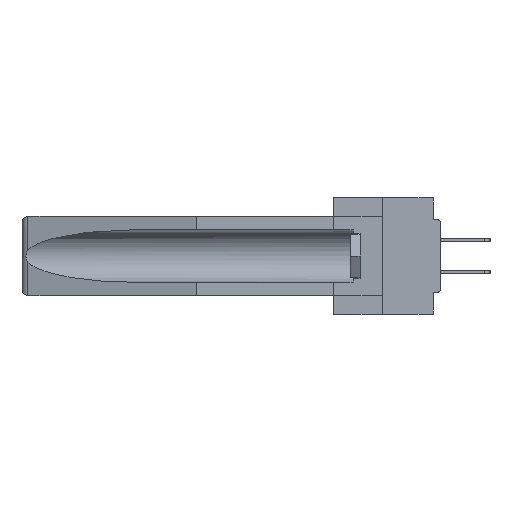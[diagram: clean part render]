
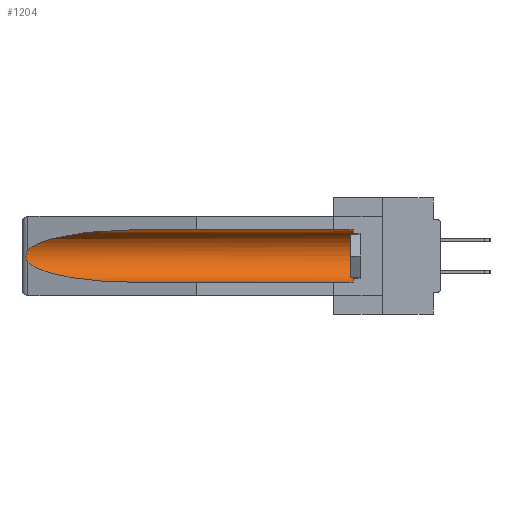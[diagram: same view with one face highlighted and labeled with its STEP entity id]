
A CAD part, left-side view. The second image highlights one B-rep face of the part: STEP entity #1204.
In plain terms, the highlighted cylindrical face has radius 2.857 mm (diameter 5.715 mm), a partial arc.
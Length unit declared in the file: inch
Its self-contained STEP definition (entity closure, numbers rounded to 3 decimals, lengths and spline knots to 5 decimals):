
#48 = CARTESIAN_POINT ( 'NONE',  ( 0.155, -0.30754, -0.1715 ) ) ;
#313 = CARTESIAN_POINT ( 'NONE',  ( 0.25451, 1.48313, -0.09465 ) ) ;
#1204 = ADVANCED_FACE ( 'NONE', ( #12092 ), #30902, .F. ) ;
#1375 = LINE ( 'NONE', #9870, #32835 ) ;
#2094 = EDGE_CURVE ( 'NONE', #26790, #12934, #27279, .T. ) ;
#2748 = B_SPLINE_CURVE_WITH_KNOTS ( 'NONE', 3,
 ( #4657, #32740, #17219, #38463, #13721, #35598, #35867, #26544, #13847, #10886 ),
 .UNSPECIFIED., .F., .F.,
 ( 4, 2, 2, 2, 4 ),
 ( 0., 0.00029, 0.00058, 0.00087, 0.00117 ),
 .UNSPECIFIED. ) ;
#2860 = CARTESIAN_POINT ( 'NONE',  ( 0.155, 0.126, -0.1715 ) ) ;
#3675 = AXIS2_PLACEMENT_3D ( 'NONE', #2860, #9345, #18841 ) ;
#4394 = CARTESIAN_POINT ( 'NONE',  ( 0.21114, 1.30732, -0.284 ) ) ;
#4505 = VERTEX_POINT ( 'NONE', #13082 ) ;
#4657 = CARTESIAN_POINT ( 'NONE',  ( 0.26537, 1.52718, -0.14972 ) ) ;
#6029 = ORIENTED_EDGE ( 'NONE', *, *, #30723, .T. ) ;
#6275 = CIRCLE ( 'NONE', #3675, 0.1125 ) ;
#6322 = CARTESIAN_POINT ( 'NONE',  ( 0.21114, 1.30732, -0.059 ) ) ;
#7328 = CARTESIAN_POINT ( 'NONE',  ( 0.26537, 1.52718, -0.14972 ) ) ;
#9345 = DIRECTION ( 'NONE',  ( 0., -1., 0. ) ) ;
#9870 = CARTESIAN_POINT ( 'NONE',  ( 0.155, -0.30754, -0.284 ) ) ;
#10499 = VERTEX_POINT ( 'NONE', #36795 ) ;
#10886 = CARTESIAN_POINT ( 'NONE',  ( 0.26537, 1.52718, -0.19328 ) ) ;
#11142 = ORIENTED_EDGE ( 'NONE', *, *, #31117, .T. ) ;
#11309 = VERTEX_POINT ( 'NONE', #14809 ) ;
#12092 = FACE_OUTER_BOUND ( 'NONE', #18877, .T. ) ;
#12934 = VERTEX_POINT ( 'NONE', #7328 ) ;
#13082 = CARTESIAN_POINT ( 'NONE',  ( 0.155, 1.07973, -0.284 ) ) ;
#13721 = CARTESIAN_POINT ( 'NONE',  ( 0.2675, 1.53308, -0.16763 ) ) ;
#13847 = CARTESIAN_POINT ( 'NONE',  ( 0.26597, 1.5296, -0.19026 ) ) ;
#14682 = EDGE_CURVE ( 'NONE', #34576, #10499, #6275, .T. ) ;
#14809 = CARTESIAN_POINT ( 'NONE',  ( 0.26537, 1.52718, -0.19328 ) ) ;
#15111 = DIRECTION ( 'NONE',  ( 0., 1., 0. ) ) ;
#17219 = CARTESIAN_POINT ( 'NONE',  ( 0.26654, 1.53092, -0.15636 ) ) ;
#18563 = LINE ( 'NONE', #27110, #19543 ) ;
#18841 = DIRECTION ( 'NONE',  ( 0., 0., 1. ) ) ;
#18877 = EDGE_LOOP ( 'NONE', ( #31115, #11142, #29495, #29835, #39743, #6029 ) ) ;
#19543 = VECTOR ( 'NONE', #27510, 39.37008 ) ;
#20088 = CARTESIAN_POINT ( 'NONE',  ( 0.155, 1.07973, -0.284 ) ) ;
#22238 = AXIS2_PLACEMENT_3D ( 'NONE', #48, #15111, #27399 ) ;
#25894 = CARTESIAN_POINT ( 'NONE',  ( 0.155, 1.07973, -0.059 ) ) ;
#26544 = CARTESIAN_POINT ( 'NONE',  ( 0.26655, 1.53094, -0.18657 ) ) ;
#26790 = VERTEX_POINT ( 'NONE', #38608 ) ;
#27110 = CARTESIAN_POINT ( 'NONE',  ( 0.155, -0.30754, -0.059 ) ) ;
#27279 =( BOUNDED_CURVE ( )  B_SPLINE_CURVE ( 3, ( #25894, #6322, #313, #40100 ),
 .UNSPECIFIED., .F., .F. ) 
 B_SPLINE_CURVE_WITH_KNOTS ( ( 4, 4 ),
 ( 4.71239, 6.08839 ),
 .UNSPECIFIED. ) 
 CURVE ( )  GEOMETRIC_REPRESENTATION_ITEM ( )  RATIONAL_B_SPLINE_CURVE ( ( 1., 0.848, 0.848, 1. ) ) 
 REPRESENTATION_ITEM ( '' )  );
#27399 = DIRECTION ( 'NONE',  ( 0., 0., 1. ) ) ;
#27510 = DIRECTION ( 'NONE',  ( 0., 1., 0. ) ) ;
#27815 = EDGE_CURVE ( 'NONE', #34576, #4505, #1375, .T. ) ;
#28001 =( BOUNDED_CURVE ( )  B_SPLINE_CURVE ( 3, ( #32465, #32605, #4394, #20088 ),
 .UNSPECIFIED., .F., .F. ) 
 B_SPLINE_CURVE_WITH_KNOTS ( ( 4, 4 ),
 ( 0.1948, 1.5708 ),
 .UNSPECIFIED. ) 
 CURVE ( )  GEOMETRIC_REPRESENTATION_ITEM ( )  RATIONAL_B_SPLINE_CURVE ( ( 1., 0.848, 0.848, 1. ) ) 
 REPRESENTATION_ITEM ( '' )  );
#29495 = ORIENTED_EDGE ( 'NONE', *, *, #31112, .T. ) ;
#29835 = ORIENTED_EDGE ( 'NONE', *, *, #27815, .F. ) ;
#30723 = EDGE_CURVE ( 'NONE', #10499, #26790, #18563, .T. ) ;
#30902 = CYLINDRICAL_SURFACE ( 'NONE', #22238, 0.1125 ) ;
#31112 = EDGE_CURVE ( 'NONE', #11309, #4505, #28001, .T. ) ;
#31115 = ORIENTED_EDGE ( 'NONE', *, *, #2094, .T. ) ;
#31117 = EDGE_CURVE ( 'NONE', #12934, #11309, #2748, .T. ) ;
#31464 = CARTESIAN_POINT ( 'NONE',  ( 0.155, 0.126, -0.284 ) ) ;
#32465 = CARTESIAN_POINT ( 'NONE',  ( 0.26537, 1.52718, -0.19328 ) ) ;
#32605 = CARTESIAN_POINT ( 'NONE',  ( 0.25451, 1.48313, -0.24835 ) ) ;
#32740 = CARTESIAN_POINT ( 'NONE',  ( 0.26597, 1.52961, -0.15275 ) ) ;
#32835 = VECTOR ( 'NONE', #37571, 39.37008 ) ;
#34576 = VERTEX_POINT ( 'NONE', #31464 ) ;
#35598 = CARTESIAN_POINT ( 'NONE',  ( 0.2675, 1.53308, -0.17534 ) ) ;
#35867 = CARTESIAN_POINT ( 'NONE',  ( 0.2673, 1.53269, -0.17917 ) ) ;
#36795 = CARTESIAN_POINT ( 'NONE',  ( 0.155, 0.126, -0.059 ) ) ;
#37571 = DIRECTION ( 'NONE',  ( 0., 1., 0. ) ) ;
#38463 = CARTESIAN_POINT ( 'NONE',  ( 0.2673, 1.5327, -0.16383 ) ) ;
#38608 = CARTESIAN_POINT ( 'NONE',  ( 0.155, 1.07973, -0.059 ) ) ;
#39743 = ORIENTED_EDGE ( 'NONE', *, *, #14682, .T. ) ;
#40100 = CARTESIAN_POINT ( 'NONE',  ( 0.26537, 1.52718, -0.14972 ) ) ;
